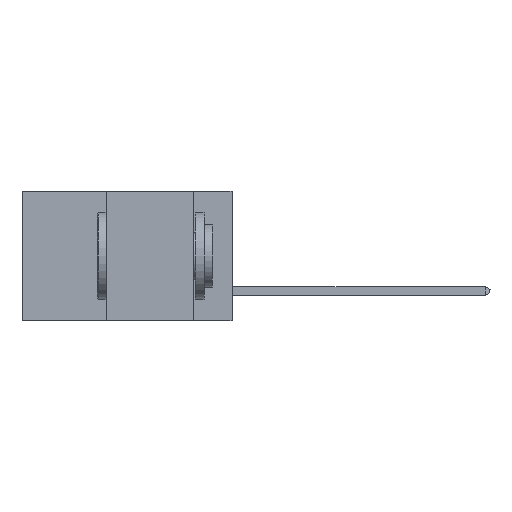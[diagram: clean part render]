
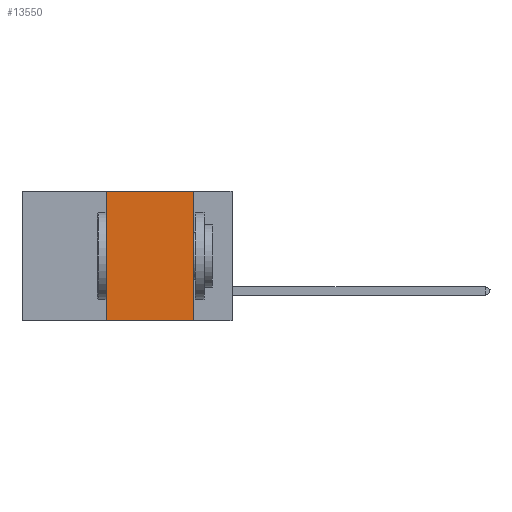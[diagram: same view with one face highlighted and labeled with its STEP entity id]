
A CAD part, left-side view. The second image highlights one B-rep face of the part: STEP entity #13550.
In plain terms, the highlighted planar face has unit normal (-1, 0, 0).
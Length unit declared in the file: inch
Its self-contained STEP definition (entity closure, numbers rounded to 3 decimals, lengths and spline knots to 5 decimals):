
#89 = VECTOR ( 'NONE', #19226, 39.37008 ) ;
#1142 = VERTEX_POINT ( 'NONE', #33370 ) ;
#1861 = PLANE ( 'NONE',  #4896 ) ;
#2320 = VECTOR ( 'NONE', #19543, 39.37008 ) ;
#3749 = CARTESIAN_POINT ( 'NONE',  ( 0., 0.11, 0. ) ) ;
#4896 = AXIS2_PLACEMENT_3D ( 'NONE', #7839, #18255, #5355 ) ;
#5057 = VECTOR ( 'NONE', #24346, 39.37008 ) ;
#5355 = DIRECTION ( 'NONE',  ( 0., 0., -1. ) ) ;
#6088 = VECTOR ( 'NONE', #17784, 39.37008 ) ;
#6199 = CARTESIAN_POINT ( 'NONE',  ( 0., 0.6, -0.37 ) ) ;
#7839 = CARTESIAN_POINT ( 'NONE',  ( 0., 0.6, 0. ) ) ;
#9207 = LINE ( 'NONE', #21430, #2320 ) ;
#11039 = LINE ( 'NONE', #6199, #89 ) ;
#13550 = ADVANCED_FACE ( 'NONE', ( #17797 ), #1861, .F. ) ;
#13827 = VERTEX_POINT ( 'NONE', #28251 ) ;
#14203 = VERTEX_POINT ( 'NONE', #29763 ) ;
#14632 = LINE ( 'NONE', #27636, #6088 ) ;
#15211 = ORIENTED_EDGE ( 'NONE', *, *, #18262, .F. ) ;
#17082 = CARTESIAN_POINT ( 'NONE',  ( 0., 0.11, 0. ) ) ;
#17522 = EDGE_CURVE ( 'NONE', #13827, #14203, #11039, .T. ) ;
#17784 = DIRECTION ( 'NONE',  ( 0., 0., 1. ) ) ;
#17797 = FACE_OUTER_BOUND ( 'NONE', #22972, .T. ) ;
#18255 = DIRECTION ( 'NONE',  ( 1., 0., 0. ) ) ;
#18262 = EDGE_CURVE ( 'NONE', #13827, #1142, #14632, .T. ) ;
#18854 = LINE ( 'NONE', #3749, #5057 ) ;
#19087 = ORIENTED_EDGE ( 'NONE', *, *, #21330, .F. ) ;
#19226 = DIRECTION ( 'NONE',  ( 0., -1., 0. ) ) ;
#19543 = DIRECTION ( 'NONE',  ( 0., -1., 0. ) ) ;
#20187 = ORIENTED_EDGE ( 'NONE', *, *, #17522, .T. ) ;
#21330 = EDGE_CURVE ( 'NONE', #32429, #14203, #18854, .T. ) ;
#21430 = CARTESIAN_POINT ( 'NONE',  ( 0., 0.6, 0. ) ) ;
#22972 = EDGE_LOOP ( 'NONE', ( #19087, #25652, #15211, #20187 ) ) ;
#24346 = DIRECTION ( 'NONE',  ( 0., 0., -1. ) ) ;
#25652 = ORIENTED_EDGE ( 'NONE', *, *, #28514, .F. ) ;
#27636 = CARTESIAN_POINT ( 'NONE',  ( 0., 0.36, 0. ) ) ;
#28251 = CARTESIAN_POINT ( 'NONE',  ( 0., 0.36, -0.37 ) ) ;
#28514 = EDGE_CURVE ( 'NONE', #1142, #32429, #9207, .T. ) ;
#29763 = CARTESIAN_POINT ( 'NONE',  ( 0., 0.11, -0.37 ) ) ;
#32429 = VERTEX_POINT ( 'NONE', #17082 ) ;
#33370 = CARTESIAN_POINT ( 'NONE',  ( 0., 0.36, 0. ) ) ;
